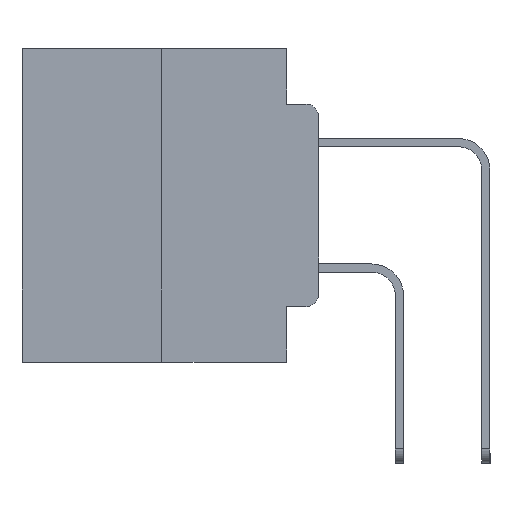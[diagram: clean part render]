
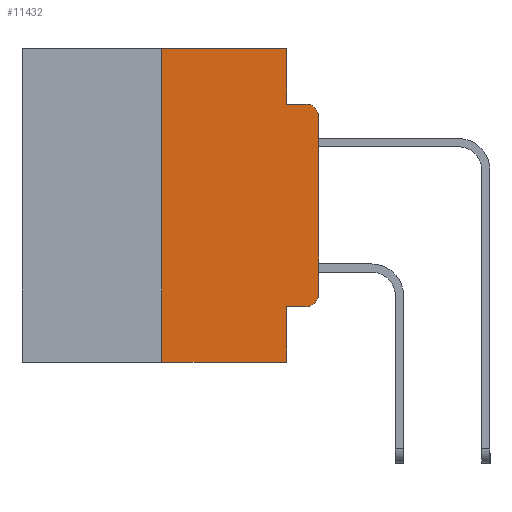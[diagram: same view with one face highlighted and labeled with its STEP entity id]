
A CAD part, left-side view. The second image highlights one B-rep face of the part: STEP entity #11432.
In plain terms, the highlighted planar face has unit normal (-1, 0, 0).
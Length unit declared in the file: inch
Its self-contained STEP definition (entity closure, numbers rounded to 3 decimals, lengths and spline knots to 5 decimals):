
#180 = AXIS2_PLACEMENT_3D ( 'NONE', #15446, #340, #15531 ) ;
#340 = DIRECTION ( 'NONE',  ( 1., 0., 0. ) ) ;
#616 = CARTESIAN_POINT ( 'NONE',  ( 0., 0., -0.3915 ) ) ;
#746 = VERTEX_POINT ( 'NONE', #2783 ) ;
#849 = ORIENTED_EDGE ( 'NONE', *, *, #14275, .F. ) ;
#1763 = CARTESIAN_POINT ( 'NONE',  ( 0., 0.051, 0. ) ) ;
#2539 = VECTOR ( 'NONE', #12618, 39.37008 ) ;
#2783 = CARTESIAN_POINT ( 'NONE',  ( 0., 0.25, 0. ) ) ;
#3202 = CARTESIAN_POINT ( 'NONE',  ( 0., 0.473, -0.5 ) ) ;
#3454 = CARTESIAN_POINT ( 'NONE',  ( 0., 0.02, -0.0885 ) ) ;
#4158 = EDGE_CURVE ( 'NONE', #26707, #13396, #10810, .T. ) ;
#4332 = CARTESIAN_POINT ( 'NONE',  ( 0., 0., -0.1085 ) ) ;
#4394 = CARTESIAN_POINT ( 'NONE',  ( 0., 0.051, 0. ) ) ;
#4454 = LINE ( 'NONE', #3202, #26305 ) ;
#4465 = CARTESIAN_POINT ( 'NONE',  ( 0., 0., 0. ) ) ;
#5026 = CARTESIAN_POINT ( 'NONE',  ( 0., 0.02, -0.4115 ) ) ;
#5273 = VECTOR ( 'NONE', #15431, 39.37008 ) ;
#5533 = EDGE_CURVE ( 'NONE', #746, #24080, #26787, .T. ) ;
#6080 = ORIENTED_EDGE ( 'NONE', *, *, #18960, .T. ) ;
#6529 = CARTESIAN_POINT ( 'NONE',  ( 0., 0.02, -0.1085 ) ) ;
#6693 = DIRECTION ( 'NONE',  ( 0., 0., 1. ) ) ;
#6943 = VERTEX_POINT ( 'NONE', #21710 ) ;
#7054 = DIRECTION ( 'NONE',  ( 0., -1., 0. ) ) ;
#7102 = ORIENTED_EDGE ( 'NONE', *, *, #27398, .T. ) ;
#7833 = ORIENTED_EDGE ( 'NONE', *, *, #24052, .T. ) ;
#8322 = DIRECTION ( 'NONE',  ( 0., 0., -1. ) ) ;
#8745 = DIRECTION ( 'NONE',  ( 0., 0., -1. ) ) ;
#9767 = LINE ( 'NONE', #1763, #2539 ) ;
#9831 = DIRECTION ( 'NONE',  ( 0., -1., 0. ) ) ;
#10213 = VERTEX_POINT ( 'NONE', #17632 ) ;
#10343 = VECTOR ( 'NONE', #6693, 39.37008 ) ;
#10810 = CIRCLE ( 'NONE', #23109, 0.02 ) ;
#10840 = EDGE_LOOP ( 'NONE', ( #23539, #7833, #11466, #26864, #18083, #849, #6080, #14125, #7102, #14448 ) ) ;
#11432 = ADVANCED_FACE ( 'NONE', ( #27017 ), #21740, .F. ) ;
#11466 = ORIENTED_EDGE ( 'NONE', *, *, #17121, .F. ) ;
#11741 = LINE ( 'NONE', #20463, #16724 ) ;
#11746 = VECTOR ( 'NONE', #16825, 39.37008 ) ;
#12494 = LINE ( 'NONE', #19069, #17475 ) ;
#12618 = DIRECTION ( 'NONE',  ( 0., 0., -1. ) ) ;
#13288 = CARTESIAN_POINT ( 'NONE',  ( 0., 0.051, -0.5 ) ) ;
#13396 = VERTEX_POINT ( 'NONE', #616 ) ;
#14125 = ORIENTED_EDGE ( 'NONE', *, *, #15682, .F. ) ;
#14227 = DIRECTION ( 'NONE',  ( 0., -1., 0. ) ) ;
#14275 = EDGE_CURVE ( 'NONE', #10213, #746, #12494, .T. ) ;
#14309 = CIRCLE ( 'NONE', #19933, 0.02 ) ;
#14448 = ORIENTED_EDGE ( 'NONE', *, *, #4158, .T. ) ;
#15154 = VERTEX_POINT ( 'NONE', #4332 ) ;
#15431 = DIRECTION ( 'NONE',  ( 0., -1., 0. ) ) ;
#15446 = CARTESIAN_POINT ( 'NONE',  ( 0., 0.473, 0. ) ) ;
#15531 = DIRECTION ( 'NONE',  ( 0., 0., -1. ) ) ;
#15682 = EDGE_CURVE ( 'NONE', #6943, #25470, #9767, .T. ) ;
#16026 = CARTESIAN_POINT ( 'NONE',  ( 0., 0.051, -0.0885 ) ) ;
#16358 = VECTOR ( 'NONE', #7054, 39.37008 ) ;
#16724 = VECTOR ( 'NONE', #14227, 39.37008 ) ;
#16825 = DIRECTION ( 'NONE',  ( 0., 0., -1. ) ) ;
#17121 = EDGE_CURVE ( 'NONE', #24369, #21165, #22209, .T. ) ;
#17475 = VECTOR ( 'NONE', #25216, 39.37008 ) ;
#17632 = CARTESIAN_POINT ( 'NONE',  ( 0., 0.25, -0.5 ) ) ;
#18083 = ORIENTED_EDGE ( 'NONE', *, *, #5533, .F. ) ;
#18960 = EDGE_CURVE ( 'NONE', #10213, #25470, #4454, .T. ) ;
#19069 = CARTESIAN_POINT ( 'NONE',  ( 0., 0.25, 0. ) ) ;
#19933 = AXIS2_PLACEMENT_3D ( 'NONE', #6529, #21328, #8745 ) ;
#20463 = CARTESIAN_POINT ( 'NONE',  ( 0., 0.051, -0.4115 ) ) ;
#21165 = VERTEX_POINT ( 'NONE', #3454 ) ;
#21286 = EDGE_CURVE ( 'NONE', #24080, #24369, #22898, .T. ) ;
#21328 = DIRECTION ( 'NONE',  ( -1., 0., 0. ) ) ;
#21551 = LINE ( 'NONE', #4465, #10343 ) ;
#21629 = CARTESIAN_POINT ( 'NONE',  ( 0., 0.051, -0.0885 ) ) ;
#21710 = CARTESIAN_POINT ( 'NONE',  ( 0., 0.051, -0.4115 ) ) ;
#21740 = PLANE ( 'NONE',  #180 ) ;
#22209 = LINE ( 'NONE', #21629, #5273 ) ;
#22657 = EDGE_CURVE ( 'NONE', #13396, #15154, #21551, .T. ) ;
#22787 = DIRECTION ( 'NONE',  ( -1., 0., 0. ) ) ;
#22898 = LINE ( 'NONE', #27206, #11746 ) ;
#23109 = AXIS2_PLACEMENT_3D ( 'NONE', #27366, #22787, #8322 ) ;
#23539 = ORIENTED_EDGE ( 'NONE', *, *, #22657, .T. ) ;
#23723 = CARTESIAN_POINT ( 'NONE',  ( 0., 0.473, 0. ) ) ;
#24052 = EDGE_CURVE ( 'NONE', #15154, #21165, #14309, .T. ) ;
#24080 = VERTEX_POINT ( 'NONE', #4394 ) ;
#24369 = VERTEX_POINT ( 'NONE', #16026 ) ;
#25216 = DIRECTION ( 'NONE',  ( 0., 0., 1. ) ) ;
#25470 = VERTEX_POINT ( 'NONE', #13288 ) ;
#26305 = VECTOR ( 'NONE', #9831, 39.37008 ) ;
#26707 = VERTEX_POINT ( 'NONE', #5026 ) ;
#26787 = LINE ( 'NONE', #23723, #16358 ) ;
#26864 = ORIENTED_EDGE ( 'NONE', *, *, #21286, .F. ) ;
#27017 = FACE_OUTER_BOUND ( 'NONE', #10840, .T. ) ;
#27206 = CARTESIAN_POINT ( 'NONE',  ( 0., 0.051, 0. ) ) ;
#27366 = CARTESIAN_POINT ( 'NONE',  ( 0., 0.02, -0.3915 ) ) ;
#27398 = EDGE_CURVE ( 'NONE', #6943, #26707, #11741, .T. ) ;
